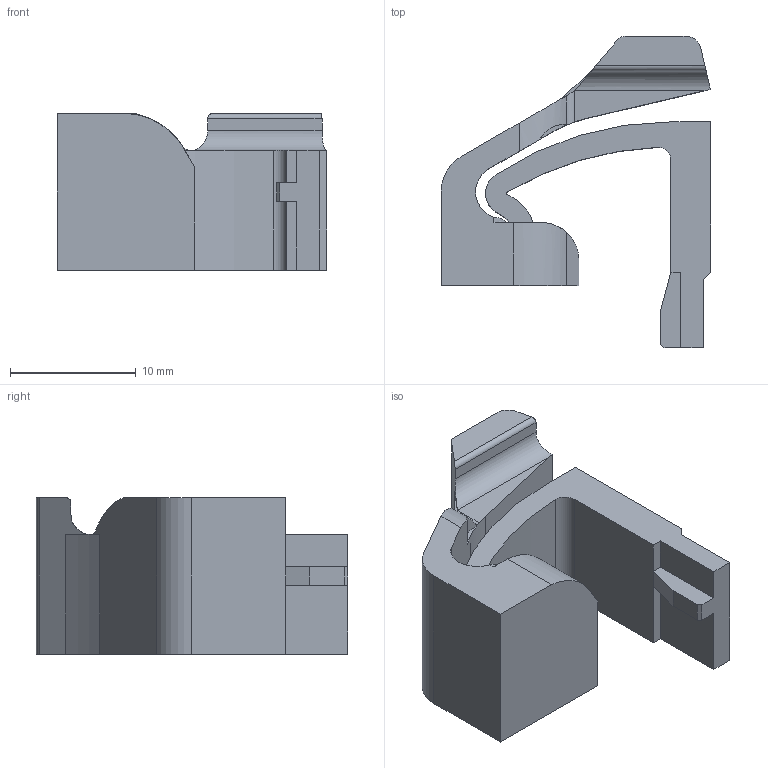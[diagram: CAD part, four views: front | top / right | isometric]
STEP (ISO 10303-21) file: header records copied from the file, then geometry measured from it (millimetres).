
FILE_DESCRIPTION(/* description */ (''),/* implementation_level */ '2;1');
FILE_NAME(/* name */ 'CB High1.stp',/* time_stamp */ '2022-11-09T21:43:35-05:00',/* author */ ('author'),/* organization */ (''),/* preprocessor_version */ 'ST-DEVELOPER v18.1',/* originating_system */ 'Autodesk Inventor 2022',/* authorisation */ '');
FILE_SCHEMA (('AUTOMOTIVE_DESIGN { 1 0 10303 214 3 1 1 }'));
Length unit declared in the file: metre
Products named in the file (1): CB High1
Bounding box: 21.42 x 24.74 x 12.45 mm (x, y, z)
Volume: 2365.3 mm3; surface area: 2134.9 mm2
Topology: 1 solids, 1 shells, 59 faces, 167 edges, 111 vertices
Faces by surface type: plane 35, cylinder 24
Entity records: 2003 total; most frequent: CARTESIAN_POINT 371, ORIENTED_EDGE 334, DIRECTION 330, EDGE_CURVE 167, LINE 114, VECTOR 114, VERTEX_POINT 110, AXIS2_PLACEMENT_3D 108
